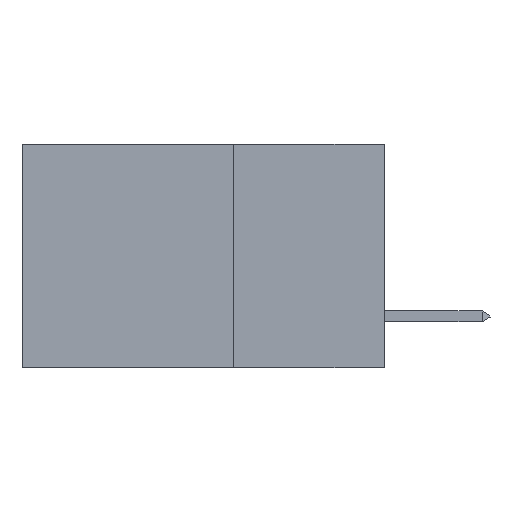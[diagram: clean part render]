
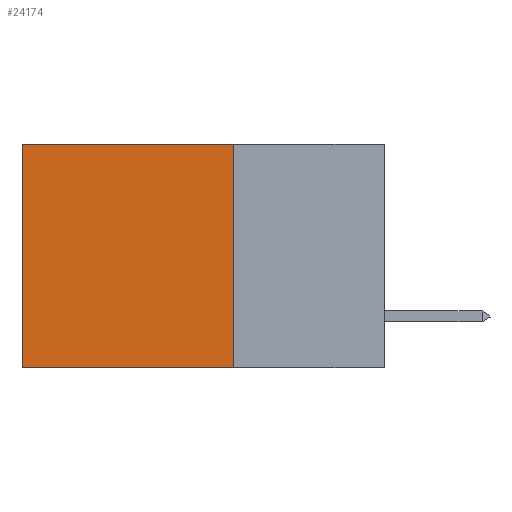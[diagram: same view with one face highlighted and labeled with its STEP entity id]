
A CAD part, left-side view. The second image highlights one B-rep face of the part: STEP entity #24174.
In plain terms, the highlighted planar face has unit normal (-1, 0, 0).
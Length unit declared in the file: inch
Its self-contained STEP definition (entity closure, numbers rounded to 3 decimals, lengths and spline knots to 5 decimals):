
#2704 = DIRECTION ( 'NONE',  ( 0., 0., -1. ) ) ;
#3009 = EDGE_CURVE ( 'NONE', #12756, #15517, #23749, .T. ) ;
#4720 = DIRECTION ( 'NONE',  ( 1., 0., 0. ) ) ;
#5028 = EDGE_LOOP ( 'NONE', ( #8198, #14490, #5036, #12161 ) ) ;
#5036 = ORIENTED_EDGE ( 'NONE', *, *, #24393, .F. ) ;
#7741 = CARTESIAN_POINT ( 'NONE',  ( 0.2875, 0.25, 0. ) ) ;
#8198 = ORIENTED_EDGE ( 'NONE', *, *, #3009, .T. ) ;
#8436 = LINE ( 'NONE', #16750, #9865 ) ;
#9448 = PLANE ( 'NONE',  #25135 ) ;
#9495 = CARTESIAN_POINT ( 'NONE',  ( 0.2875, 0.6, 0. ) ) ;
#9664 = LINE ( 'NONE', #18491, #18259 ) ;
#9865 = VECTOR ( 'NONE', #10047, 39.37008 ) ;
#10047 = DIRECTION ( 'NONE',  ( 0., 0., -1. ) ) ;
#11843 = CARTESIAN_POINT ( 'NONE',  ( 0.2875, 0.25, 0. ) ) ;
#11966 = DIRECTION ( 'NONE',  ( 0., 1., 0. ) ) ;
#12161 = ORIENTED_EDGE ( 'NONE', *, *, #28398, .T. ) ;
#12756 = VERTEX_POINT ( 'NONE', #9495 ) ;
#12760 = VERTEX_POINT ( 'NONE', #27870 ) ;
#14210 = VERTEX_POINT ( 'NONE', #19464 ) ;
#14490 = ORIENTED_EDGE ( 'NONE', *, *, #16463, .F. ) ;
#14723 = CARTESIAN_POINT ( 'NONE',  ( 0.2875, 0.6, -0.37 ) ) ;
#15517 = VERTEX_POINT ( 'NONE', #14723 ) ;
#16463 = EDGE_CURVE ( 'NONE', #12760, #15517, #9664, .T. ) ;
#16750 = CARTESIAN_POINT ( 'NONE',  ( 0.2875, 0.25, 0. ) ) ;
#18259 = VECTOR ( 'NONE', #11966, 39.37008 ) ;
#18491 = CARTESIAN_POINT ( 'NONE',  ( 0.2875, 0.25, -0.37 ) ) ;
#19464 = CARTESIAN_POINT ( 'NONE',  ( 0.2875, 0.25, 0. ) ) ;
#20857 = VECTOR ( 'NONE', #29659, 39.37008 ) ;
#23749 = LINE ( 'NONE', #27319, #20857 ) ;
#24174 = ADVANCED_FACE ( 'NONE', ( #28913 ), #9448, .F. ) ;
#24181 = DIRECTION ( 'NONE',  ( 0., 1., 0. ) ) ;
#24393 = EDGE_CURVE ( 'NONE', #14210, #12760, #8436, .T. ) ;
#25135 = AXIS2_PLACEMENT_3D ( 'NONE', #11843, #4720, #2704 ) ;
#25790 = LINE ( 'NONE', #7741, #27951 ) ;
#27319 = CARTESIAN_POINT ( 'NONE',  ( 0.2875, 0.6, 0. ) ) ;
#27870 = CARTESIAN_POINT ( 'NONE',  ( 0.2875, 0.25, -0.37 ) ) ;
#27951 = VECTOR ( 'NONE', #24181, 39.37008 ) ;
#28398 = EDGE_CURVE ( 'NONE', #14210, #12756, #25790, .T. ) ;
#28913 = FACE_OUTER_BOUND ( 'NONE', #5028, .T. ) ;
#29659 = DIRECTION ( 'NONE',  ( 0., 0., -1. ) ) ;
